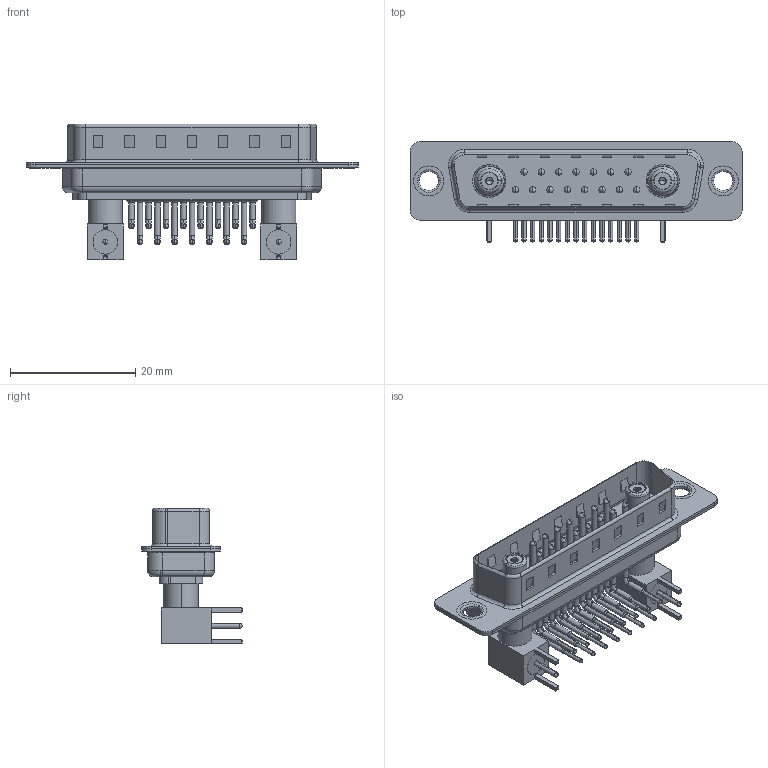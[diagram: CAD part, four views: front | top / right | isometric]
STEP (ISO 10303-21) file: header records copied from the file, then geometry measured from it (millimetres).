
FILE_DESCRIPTION (( 'STEP AP203' ), '1' );
FILE_NAME ('629-17W2240-7N1.STEP', '2022-05-10T11:47:37', ( '' ), ( '' ), 'SwSTEP 2.0', 'SolidWorks 2020', '' );
FILE_SCHEMA (( 'CONFIG_CONTROL_DESIGN' ));
Length unit declared in the file: millimetre
Products named in the file (16): Co-Ax Jack Assy_RA; 629Combo Thru Hole Rivet; 629Combo Contact Row 2; 629Combo Shell Front_25 Contacts; Co-Ax Jack_RA PC Tail; Insulator Socket 2; 629Combo Shell Rear_25 Contacts; Insulator Socket; 629Combo Housing_17W2; Locking Collar; Insulator RA Pin; 629Combo Contact Row 1; RA Back Shell; Socket_RA; 629-17W2240-7N1
Assembly tree (36 placements, depth 3):
  629-17W2240-7N1
    629Combo Housing_17W2
    629Combo Shell Rear_25 Contacts
    629Combo Shell Front_25 Contacts
    629Combo Thru Hole Rivet  x2
    Co-Ax Jack Assy_RA
      Co-Ax Jack_RA PC Tail
      Insulator Socket
      Insulator Socket 2
      Locking Collar
      Socket_RA
      RA Back Shell
      Insulator RA Pin
    Co-Ax Jack Assy_RA
      Co-Ax Jack_RA PC Tail
      Insulator Socket
      Insulator Socket 2
      Locking Collar
      Socket_RA
      RA Back Shell
      Insulator RA Pin
    629Combo Contact Row 1  x7
    629Combo Contact Row 2  x8
Bounding box: 53.05 x 16 x 21.71 mm (x, y, z)
Volume: 3331.5 mm3; surface area: 9019.3 mm2
Topology: 34 solids, 34 shells, 2304 faces, 6229 edges, 4016 vertices
Faces by surface type: plane 1245, cylinder 795, cone 98, bspline 92, torus 70, sphere 4
Entity records: 27153 total; most frequent: CARTESIAN_POINT 4622, DIRECTION 4465, ORIENTED_EDGE 4056, EDGE_CURVE 2028, AXIS2_PLACEMENT_3D 1631, VERTEX_POINT 1303, LINE 1203, VECTOR 1203
